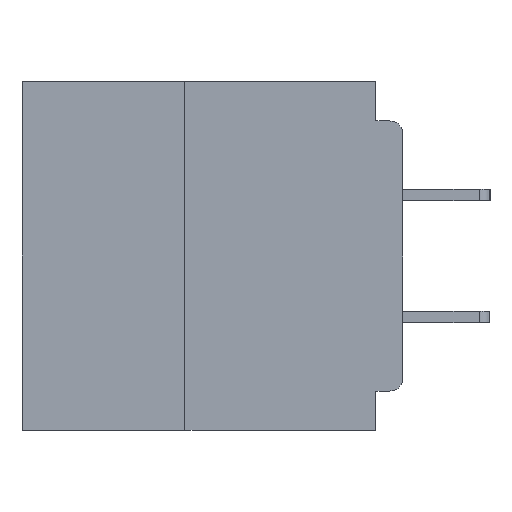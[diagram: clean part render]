
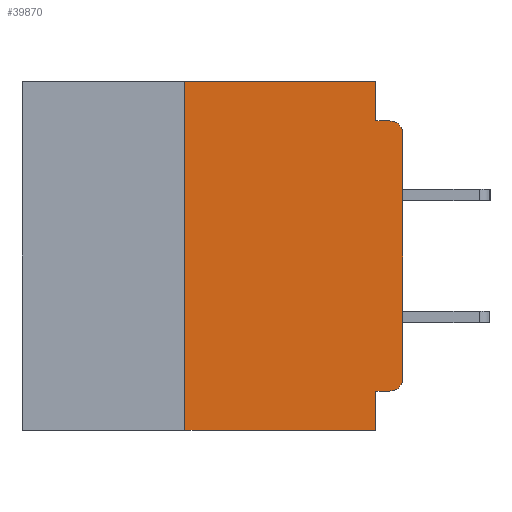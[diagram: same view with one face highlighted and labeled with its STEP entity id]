
A CAD part, left-side view. The second image highlights one B-rep face of the part: STEP entity #39870.
In plain terms, the highlighted planar face has unit normal (-1, 0, 0).
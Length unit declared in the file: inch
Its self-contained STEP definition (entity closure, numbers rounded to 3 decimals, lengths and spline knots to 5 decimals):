
#213 = VERTEX_POINT ( 'NONE', #39833 ) ;
#294 = CARTESIAN_POINT ( 'NONE',  ( 0., 0.031, -0.355 ) ) ;
#774 = DIRECTION ( 'NONE',  ( 0., -1., 0. ) ) ;
#1910 = CARTESIAN_POINT ( 'NONE',  ( 0., 0.031, 0. ) ) ;
#2667 = FACE_OUTER_BOUND ( 'NONE', #20001, .T. ) ;
#2720 = DIRECTION ( 'NONE',  ( 0., 0., -1. ) ) ;
#3247 = EDGE_CURVE ( 'NONE', #21646, #10333, #22494, .T. ) ;
#5491 = ORIENTED_EDGE ( 'NONE', *, *, #17705, .F. ) ;
#5750 = AXIS2_PLACEMENT_3D ( 'NONE', #9860, #31655, #12994 ) ;
#6235 = CARTESIAN_POINT ( 'NONE',  ( 0., 0.437, 0. ) ) ;
#6584 = VECTOR ( 'NONE', #14339, 39.37008 ) ;
#6810 = EDGE_CURVE ( 'NONE', #11812, #23406, #18352, .T. ) ;
#6908 = VERTEX_POINT ( 'NONE', #24146 ) ;
#6974 = DIRECTION ( 'NONE',  ( -1., 0., 0. ) ) ;
#7954 = CARTESIAN_POINT ( 'NONE',  ( 0., 0.25, -0.4 ) ) ;
#8008 = DIRECTION ( 'NONE',  ( 0., 0., 1. ) ) ;
#8168 = EDGE_CURVE ( 'NONE', #11812, #13883, #15274, .T. ) ;
#8247 = CARTESIAN_POINT ( 'NONE',  ( 0., 0.015, -0.045 ) ) ;
#8255 = DIRECTION ( 'NONE',  ( 0., 0., -1. ) ) ;
#8446 = CARTESIAN_POINT ( 'NONE',  ( 0., 0.437, -0.4 ) ) ;
#9343 = DIRECTION ( 'NONE',  ( 0., -1., 0. ) ) ;
#9530 = CARTESIAN_POINT ( 'NONE',  ( 0., 0., -0.06 ) ) ;
#9860 = CARTESIAN_POINT ( 'NONE',  ( 0., 0.015, -0.06 ) ) ;
#10333 = VERTEX_POINT ( 'NONE', #28516 ) ;
#10357 = ORIENTED_EDGE ( 'NONE', *, *, #20605, .F. ) ;
#10522 = CARTESIAN_POINT ( 'NONE',  ( 0., 0.031, 0. ) ) ;
#11176 = CARTESIAN_POINT ( 'NONE',  ( 0., 0., -0.355 ) ) ;
#11395 = LINE ( 'NONE', #16518, #26094 ) ;
#11424 = DIRECTION ( 'NONE',  ( 0., -1., 0. ) ) ;
#11812 = VERTEX_POINT ( 'NONE', #7954 ) ;
#11845 = ORIENTED_EDGE ( 'NONE', *, *, #23983, .T. ) ;
#12994 = DIRECTION ( 'NONE',  ( 0., 0., -1. ) ) ;
#13168 = VECTOR ( 'NONE', #9343, 39.37008 ) ;
#13260 = ORIENTED_EDGE ( 'NONE', *, *, #33497, .T. ) ;
#13360 = CARTESIAN_POINT ( 'NONE',  ( 0., 0., -0.045 ) ) ;
#13883 = VERTEX_POINT ( 'NONE', #15788 ) ;
#14146 = VECTOR ( 'NONE', #2720, 39.37008 ) ;
#14216 = VERTEX_POINT ( 'NONE', #8247 ) ;
#14339 = DIRECTION ( 'NONE',  ( 0., 1., 0. ) ) ;
#15165 = VERTEX_POINT ( 'NONE', #9530 ) ;
#15274 = LINE ( 'NONE', #8446, #29882 ) ;
#15788 = CARTESIAN_POINT ( 'NONE',  ( 0., 0.031, -0.4 ) ) ;
#16518 = CARTESIAN_POINT ( 'NONE',  ( 0., 0., 0. ) ) ;
#17705 = EDGE_CURVE ( 'NONE', #23406, #21646, #37966, .T. ) ;
#18352 = LINE ( 'NONE', #38967, #32879 ) ;
#20001 = EDGE_LOOP ( 'NONE', ( #11845, #13260, #34663, #28428, #5491, #22128, #24099, #10357, #21655, #23622 ) ) ;
#20586 = PLANE ( 'NONE',  #34542 ) ;
#20605 = EDGE_CURVE ( 'NONE', #36293, #13883, #20808, .T. ) ;
#20724 = CARTESIAN_POINT ( 'NONE',  ( 0., 0.437, 0. ) ) ;
#20808 = LINE ( 'NONE', #27608, #28064 ) ;
#21646 = VERTEX_POINT ( 'NONE', #10522 ) ;
#21655 = ORIENTED_EDGE ( 'NONE', *, *, #23639, .F. ) ;
#22128 = ORIENTED_EDGE ( 'NONE', *, *, #6810, .F. ) ;
#22134 = DIRECTION ( 'NONE',  ( 0., 0., 1. ) ) ;
#22448 = CARTESIAN_POINT ( 'NONE',  ( 0., 0.25, 0. ) ) ;
#22494 = LINE ( 'NONE', #1910, #14146 ) ;
#23319 = VECTOR ( 'NONE', #774, 39.37008 ) ;
#23406 = VERTEX_POINT ( 'NONE', #22448 ) ;
#23622 = ORIENTED_EDGE ( 'NONE', *, *, #34131, .T. ) ;
#23639 = EDGE_CURVE ( 'NONE', #6908, #36293, #31403, .T. ) ;
#23983 = EDGE_CURVE ( 'NONE', #213, #15165, #11395, .T. ) ;
#24099 = ORIENTED_EDGE ( 'NONE', *, *, #8168, .T. ) ;
#24146 = CARTESIAN_POINT ( 'NONE',  ( 0., 0.015, -0.355 ) ) ;
#24283 = LINE ( 'NONE', #13360, #23319 ) ;
#24445 = CIRCLE ( 'NONE', #5750, 0.015 ) ;
#25684 = CARTESIAN_POINT ( 'NONE',  ( 0., 0.015, -0.34 ) ) ;
#26094 = VECTOR ( 'NONE', #22134, 39.37008 ) ;
#26960 = DIRECTION ( 'NONE',  ( 1., 0., 0. ) ) ;
#27608 = CARTESIAN_POINT ( 'NONE',  ( 0., 0.031, -0.4 ) ) ;
#28064 = VECTOR ( 'NONE', #30697, 39.37008 ) ;
#28428 = ORIENTED_EDGE ( 'NONE', *, *, #3247, .F. ) ;
#28516 = CARTESIAN_POINT ( 'NONE',  ( 0., 0.031, -0.045 ) ) ;
#28779 = DIRECTION ( 'NONE',  ( 0., 0., -1. ) ) ;
#29257 = AXIS2_PLACEMENT_3D ( 'NONE', #25684, #6974, #28779 ) ;
#29882 = VECTOR ( 'NONE', #11424, 39.37008 ) ;
#30697 = DIRECTION ( 'NONE',  ( 0., 0., -1. ) ) ;
#31403 = LINE ( 'NONE', #11176, #6584 ) ;
#31655 = DIRECTION ( 'NONE',  ( -1., 0., 0. ) ) ;
#32879 = VECTOR ( 'NONE', #8008, 39.37008 ) ;
#33497 = EDGE_CURVE ( 'NONE', #15165, #14216, #24445, .T. ) ;
#34131 = EDGE_CURVE ( 'NONE', #6908, #213, #34386, .T. ) ;
#34179 = EDGE_CURVE ( 'NONE', #10333, #14216, #24283, .T. ) ;
#34386 = CIRCLE ( 'NONE', #29257, 0.015 ) ;
#34542 = AXIS2_PLACEMENT_3D ( 'NONE', #20724, #26960, #8255 ) ;
#34663 = ORIENTED_EDGE ( 'NONE', *, *, #34179, .F. ) ;
#36293 = VERTEX_POINT ( 'NONE', #294 ) ;
#37966 = LINE ( 'NONE', #6235, #13168 ) ;
#38967 = CARTESIAN_POINT ( 'NONE',  ( 0., 0.25, -0.4 ) ) ;
#39833 = CARTESIAN_POINT ( 'NONE',  ( 0., 0., -0.34 ) ) ;
#39870 = ADVANCED_FACE ( 'NONE', ( #2667 ), #20586, .F. ) ;
